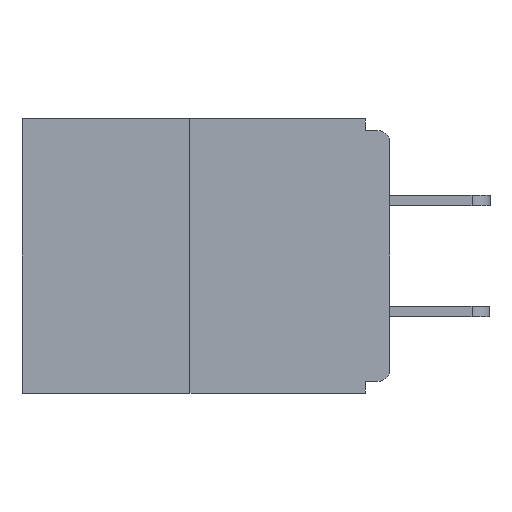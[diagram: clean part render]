
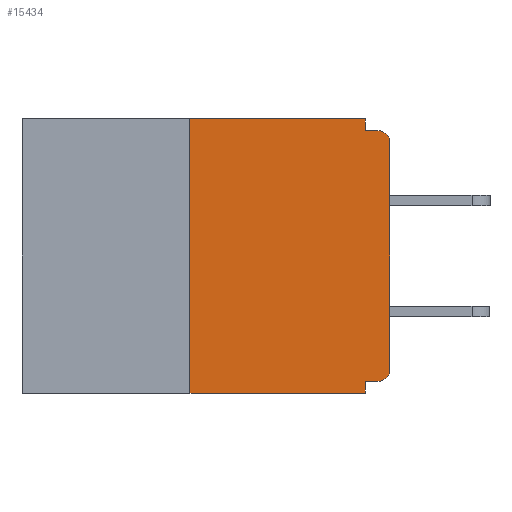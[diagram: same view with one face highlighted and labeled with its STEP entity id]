
A CAD part, left-side view. The second image highlights one B-rep face of the part: STEP entity #15434.
In plain terms, the highlighted planar face has unit normal (-1, 0, 0).
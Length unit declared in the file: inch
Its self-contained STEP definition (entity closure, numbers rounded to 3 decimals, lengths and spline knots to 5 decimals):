
#261 = DIRECTION ( 'NONE',  ( -1., 0., 0. ) ) ;
#400 = CARTESIAN_POINT ( 'NONE',  ( 0., 0., -0.03 ) ) ;
#428 = ORIENTED_EDGE ( 'NONE', *, *, #7161, .T. ) ;
#591 = CARTESIAN_POINT ( 'NONE',  ( 0., 0.25, -0.343 ) ) ;
#1213 = DIRECTION ( 'NONE',  ( -1., 0., 0. ) ) ;
#1368 = VECTOR ( 'NONE', #2511, 39.37008 ) ;
#1483 = DIRECTION ( 'NONE',  ( 0., 1., 0. ) ) ;
#1897 = EDGE_CURVE ( 'NONE', #4989, #7643, #8840, .T. ) ;
#2245 = DIRECTION ( 'NONE',  ( 0., -1., 0. ) ) ;
#2393 = PLANE ( 'NONE',  #10782 ) ;
#2464 = CARTESIAN_POINT ( 'NONE',  ( 0., 0., -0.313 ) ) ;
#2511 = DIRECTION ( 'NONE',  ( 0., 0., 1. ) ) ;
#2878 = DIRECTION ( 'NONE',  ( 0., 0., 1. ) ) ;
#2963 = LINE ( 'NONE', #8942, #4100 ) ;
#3027 = ORIENTED_EDGE ( 'NONE', *, *, #1897, .F. ) ;
#3221 = CARTESIAN_POINT ( 'NONE',  ( 0., 0.031, 0. ) ) ;
#3689 = DIRECTION ( 'NONE',  ( 1., 0., 0. ) ) ;
#3773 = CARTESIAN_POINT ( 'NONE',  ( 0., 0.031, 0. ) ) ;
#3954 = EDGE_LOOP ( 'NONE', ( #3027, #7440, #10558, #4970, #6372, #15695, #14171, #428, #5050, #9847 ) ) ;
#4100 = VECTOR ( 'NONE', #1483, 39.37008 ) ;
#4151 = CARTESIAN_POINT ( 'NONE',  ( 0., 0.25, 0. ) ) ;
#4604 = VERTEX_POINT ( 'NONE', #591 ) ;
#4683 = FACE_OUTER_BOUND ( 'NONE', #3954, .T. ) ;
#4807 = CARTESIAN_POINT ( 'NONE',  ( 0., 0.031, -0.343 ) ) ;
#4970 = ORIENTED_EDGE ( 'NONE', *, *, #13611, .F. ) ;
#4989 = VERTEX_POINT ( 'NONE', #7684 ) ;
#5050 = ORIENTED_EDGE ( 'NONE', *, *, #9426, .F. ) ;
#5432 = AXIS2_PLACEMENT_3D ( 'NONE', #8642, #1213, #9901 ) ;
#5511 = EDGE_CURVE ( 'NONE', #5722, #11995, #2963, .T. ) ;
#5528 = AXIS2_PLACEMENT_3D ( 'NONE', #10290, #261, #11518 ) ;
#5564 = CARTESIAN_POINT ( 'NONE',  ( 0., 0.015, -0.328 ) ) ;
#5722 = VERTEX_POINT ( 'NONE', #5564 ) ;
#5987 = CARTESIAN_POINT ( 'NONE',  ( 0., 0., -0.015 ) ) ;
#6372 = ORIENTED_EDGE ( 'NONE', *, *, #5511, .F. ) ;
#7161 = EDGE_CURVE ( 'NONE', #8007, #8879, #11849, .T. ) ;
#7217 = LINE ( 'NONE', #15669, #9751 ) ;
#7440 = ORIENTED_EDGE ( 'NONE', *, *, #8400, .F. ) ;
#7456 = VECTOR ( 'NONE', #2245, 39.37008 ) ;
#7643 = VERTEX_POINT ( 'NONE', #3773 ) ;
#7684 = CARTESIAN_POINT ( 'NONE',  ( 0., 0.25, 0. ) ) ;
#7914 = CARTESIAN_POINT ( 'NONE',  ( 0., 0.031, -0.015 ) ) ;
#8007 = VERTEX_POINT ( 'NONE', #400 ) ;
#8010 = DIRECTION ( 'NONE',  ( 0., -1., 0. ) ) ;
#8400 = EDGE_CURVE ( 'NONE', #4604, #4989, #15627, .T. ) ;
#8642 = CARTESIAN_POINT ( 'NONE',  ( 0., 0.015, -0.313 ) ) ;
#8791 = CARTESIAN_POINT ( 'NONE',  ( 0., 0.46, 0. ) ) ;
#8840 = LINE ( 'NONE', #8791, #13644 ) ;
#8879 = VERTEX_POINT ( 'NONE', #11332 ) ;
#8942 = CARTESIAN_POINT ( 'NONE',  ( 0., 0., -0.328 ) ) ;
#9197 = VECTOR ( 'NONE', #15512, 39.37008 ) ;
#9426 = EDGE_CURVE ( 'NONE', #13392, #8879, #15014, .T. ) ;
#9751 = VECTOR ( 'NONE', #12040, 39.37008 ) ;
#9784 = EDGE_CURVE ( 'NONE', #7643, #13392, #14560, .T. ) ;
#9847 = ORIENTED_EDGE ( 'NONE', *, *, #9784, .F. ) ;
#9901 = DIRECTION ( 'NONE',  ( 0., 0., -1. ) ) ;
#10115 = LINE ( 'NONE', #13809, #1368 ) ;
#10290 = CARTESIAN_POINT ( 'NONE',  ( 0., 0.015, -0.03 ) ) ;
#10558 = ORIENTED_EDGE ( 'NONE', *, *, #10617, .T. ) ;
#10617 = EDGE_CURVE ( 'NONE', #4604, #13075, #7217, .T. ) ;
#10782 = AXIS2_PLACEMENT_3D ( 'NONE', #12268, #3689, #12213 ) ;
#11198 = DIRECTION ( 'NONE',  ( 0., 0., -1. ) ) ;
#11332 = CARTESIAN_POINT ( 'NONE',  ( 0., 0.015, -0.015 ) ) ;
#11410 = CARTESIAN_POINT ( 'NONE',  ( 0., 0.031, -0.328 ) ) ;
#11518 = DIRECTION ( 'NONE',  ( 0., 0., -1. ) ) ;
#11849 = CIRCLE ( 'NONE', #5528, 0.015 ) ;
#11865 = EDGE_CURVE ( 'NONE', #14053, #8007, #10115, .T. ) ;
#11995 = VERTEX_POINT ( 'NONE', #11410 ) ;
#12040 = DIRECTION ( 'NONE',  ( 0., -1., 0. ) ) ;
#12172 = VECTOR ( 'NONE', #11198, 39.37008 ) ;
#12213 = DIRECTION ( 'NONE',  ( 0., 0., -1. ) ) ;
#12268 = CARTESIAN_POINT ( 'NONE',  ( 0., 0.46, 0. ) ) ;
#12387 = VECTOR ( 'NONE', #2878, 39.37008 ) ;
#12477 = CARTESIAN_POINT ( 'NONE',  ( 0., 0.031, -0.343 ) ) ;
#12748 = LINE ( 'NONE', #12477, #12172 ) ;
#13075 = VERTEX_POINT ( 'NONE', #4807 ) ;
#13392 = VERTEX_POINT ( 'NONE', #7914 ) ;
#13611 = EDGE_CURVE ( 'NONE', #11995, #13075, #12748, .T. ) ;
#13644 = VECTOR ( 'NONE', #8010, 39.37008 ) ;
#13809 = CARTESIAN_POINT ( 'NONE',  ( 0., 0., 0. ) ) ;
#14053 = VERTEX_POINT ( 'NONE', #2464 ) ;
#14171 = ORIENTED_EDGE ( 'NONE', *, *, #11865, .T. ) ;
#14560 = LINE ( 'NONE', #3221, #9197 ) ;
#14905 = EDGE_CURVE ( 'NONE', #5722, #14053, #15570, .T. ) ;
#15014 = LINE ( 'NONE', #5987, #7456 ) ;
#15434 = ADVANCED_FACE ( 'NONE', ( #4683 ), #2393, .F. ) ;
#15512 = DIRECTION ( 'NONE',  ( 0., 0., -1. ) ) ;
#15570 = CIRCLE ( 'NONE', #5432, 0.015 ) ;
#15627 = LINE ( 'NONE', #4151, #12387 ) ;
#15669 = CARTESIAN_POINT ( 'NONE',  ( 0., 0.46, -0.343 ) ) ;
#15695 = ORIENTED_EDGE ( 'NONE', *, *, #14905, .T. ) ;
